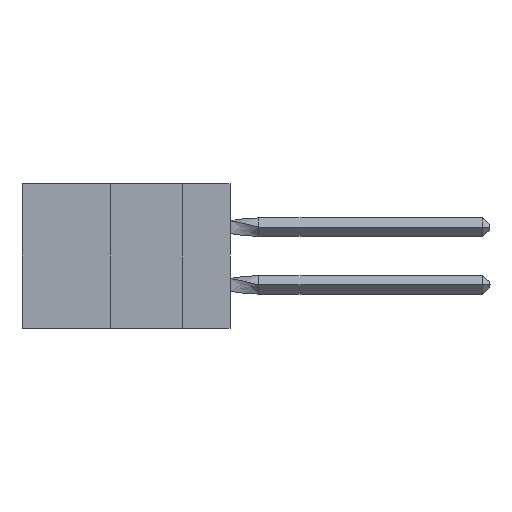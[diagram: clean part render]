
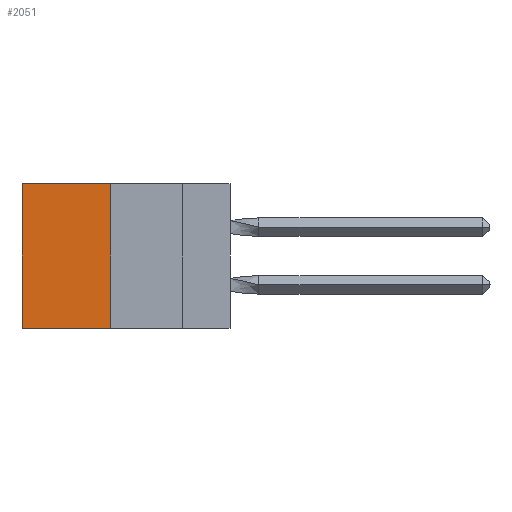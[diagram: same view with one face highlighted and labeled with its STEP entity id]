
A CAD part, left-side view. The second image highlights one B-rep face of the part: STEP entity #2051.
In plain terms, the highlighted planar face has unit normal (-1, 0, 0).
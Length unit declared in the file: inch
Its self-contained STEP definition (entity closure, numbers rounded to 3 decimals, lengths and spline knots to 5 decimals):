
#356 = VECTOR ( 'NONE', #23288, 39.37008 ) ;
#989 = VECTOR ( 'NONE', #23064, 39.37008 ) ;
#1683 = CARTESIAN_POINT ( 'NONE',  ( 0.305, 0.413, -0.5 ) ) ;
#2051 = ADVANCED_FACE ( 'NONE', ( #3254 ), #19345, .F. ) ;
#2312 = CARTESIAN_POINT ( 'NONE',  ( 0.305, 0.413, 0. ) ) ;
#2670 = CARTESIAN_POINT ( 'NONE',  ( 0.305, 0.72, 0. ) ) ;
#2696 = DIRECTION ( 'NONE',  ( 1., 0., 0. ) ) ;
#2759 = ORIENTED_EDGE ( 'NONE', *, *, #17196, .T. ) ;
#3195 = CARTESIAN_POINT ( 'NONE',  ( 0.305, 0.413, -0.5 ) ) ;
#3254 = FACE_OUTER_BOUND ( 'NONE', #20017, .T. ) ;
#3348 = DIRECTION ( 'NONE',  ( 0., 1., 0. ) ) ;
#3855 = LINE ( 'NONE', #6806, #17828 ) ;
#5027 = VECTOR ( 'NONE', #5148, 39.37008 ) ;
#5148 = DIRECTION ( 'NONE',  ( 0., 0., -1. ) ) ;
#5534 = VERTEX_POINT ( 'NONE', #2670 ) ;
#5968 = LINE ( 'NONE', #2312, #989 ) ;
#6339 = ORIENTED_EDGE ( 'NONE', *, *, #15795, .T. ) ;
#6806 = CARTESIAN_POINT ( 'NONE',  ( 0.305, 0.413, -0.5 ) ) ;
#7996 = EDGE_CURVE ( 'NONE', #10992, #12661, #3855, .T. ) ;
#8067 = EDGE_CURVE ( 'NONE', #17434, #10992, #14604, .T. ) ;
#8950 = ORIENTED_EDGE ( 'NONE', *, *, #7996, .F. ) ;
#9477 = ORIENTED_EDGE ( 'NONE', *, *, #8067, .F. ) ;
#10992 = VERTEX_POINT ( 'NONE', #1683 ) ;
#11736 = DIRECTION ( 'NONE',  ( 0., 0., -1. ) ) ;
#12661 = VERTEX_POINT ( 'NONE', #17100 ) ;
#14576 = AXIS2_PLACEMENT_3D ( 'NONE', #21059, #2696, #11736 ) ;
#14604 = LINE ( 'NONE', #3195, #5027 ) ;
#15795 = EDGE_CURVE ( 'NONE', #5534, #12661, #20722, .T. ) ;
#17100 = CARTESIAN_POINT ( 'NONE',  ( 0.305, 0.72, -0.5 ) ) ;
#17196 = EDGE_CURVE ( 'NONE', #17434, #5534, #5968, .T. ) ;
#17434 = VERTEX_POINT ( 'NONE', #23681 ) ;
#17828 = VECTOR ( 'NONE', #3348, 39.37008 ) ;
#19345 = PLANE ( 'NONE',  #14576 ) ;
#20017 = EDGE_LOOP ( 'NONE', ( #6339, #8950, #9477, #2759 ) ) ;
#20722 = LINE ( 'NONE', #23060, #356 ) ;
#21059 = CARTESIAN_POINT ( 'NONE',  ( 0.305, 0.413, -0.5 ) ) ;
#23060 = CARTESIAN_POINT ( 'NONE',  ( 0.305, 0.72, -0.5 ) ) ;
#23064 = DIRECTION ( 'NONE',  ( 0., 1., 0. ) ) ;
#23288 = DIRECTION ( 'NONE',  ( 0., 0., -1. ) ) ;
#23681 = CARTESIAN_POINT ( 'NONE',  ( 0.305, 0.413, 0. ) ) ;
